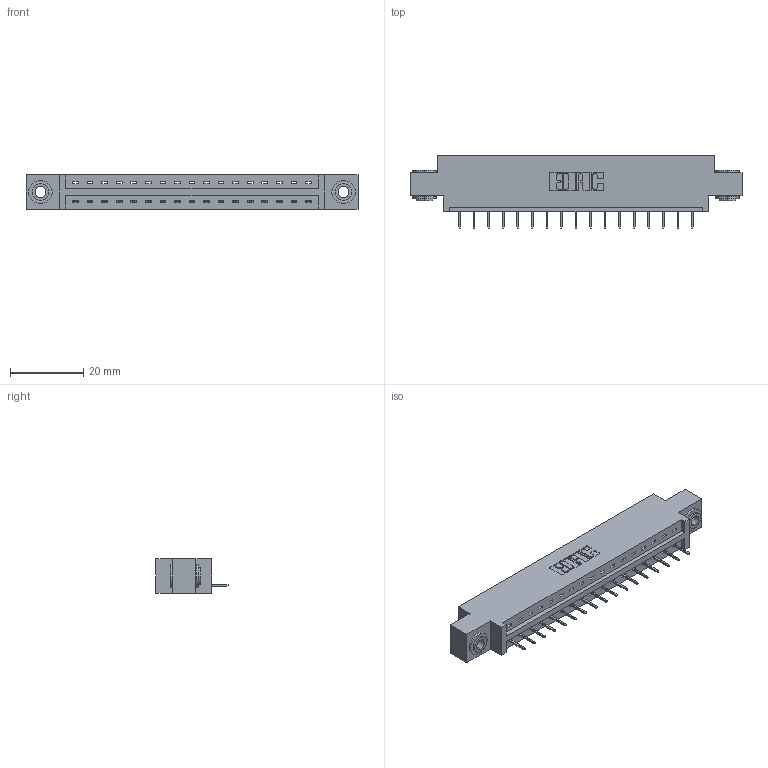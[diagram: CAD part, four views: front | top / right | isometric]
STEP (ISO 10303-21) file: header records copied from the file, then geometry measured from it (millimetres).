
FILE_DESCRIPTION (( 'STEP AP203' ), '1' );
FILE_NAME ('387-017-524-603.STEP', '2018-09-12T03:56:35', ( '' ), ( '' ), 'SwSTEP 2.0', 'SolidWorks 2016', '' );
FILE_SCHEMA (( 'CONFIG_CONTROL_DESIGN' ));
Length unit declared in the file: inch
Products named in the file (4): 345-292-001_345-293-124; 345-250-002_345-250-002-102; 387-017-524-603; 337 Part_0.170 Offset - 0.156 Dia-TH
Assembly tree (20 placements, depth 2):
  387-017-524-603
    337 Part_0.170 Offset - 0.156 Dia-TH
    345-292-001_345-293-124  x17
    345-250-002_345-250-002-102  x2
Bounding box: 90.37 x 19.69 x 9.4 mm (x, y, z)
Volume: 8914.7 mm3; surface area: 9166.2 mm2
Topology: 20 solids, 20 shells, 1278 faces, 3663 edges, 2370 vertices
Faces by surface type: plane 968, cylinder 302, cone 8
Entity records: 16726 total; most frequent: CARTESIAN_POINT 2888, ORIENTED_EDGE 2834, DIRECTION 2517, EDGE_CURVE 1417, LINE 1269, VECTOR 1269, VERTEX_POINT 938, AXIS2_PLACEMENT_3D 624
